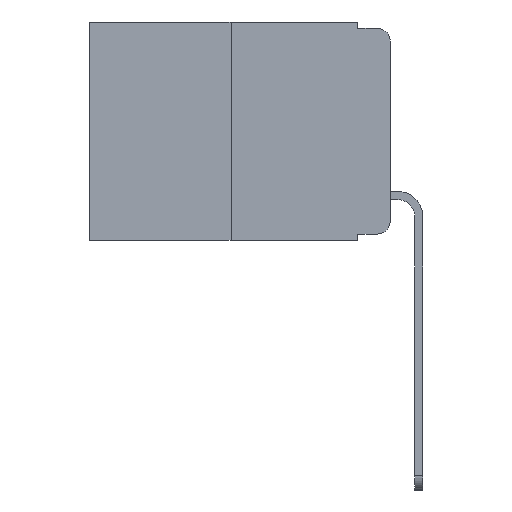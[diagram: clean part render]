
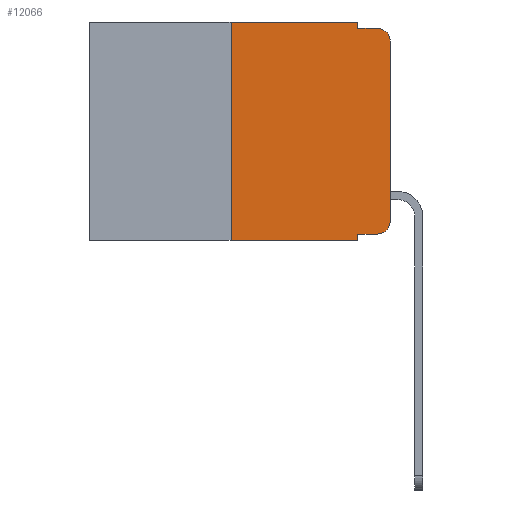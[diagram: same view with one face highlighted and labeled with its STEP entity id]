
A CAD part, left-side view. The second image highlights one B-rep face of the part: STEP entity #12066.
In plain terms, the highlighted planar face has unit normal (-1, 0, 0).
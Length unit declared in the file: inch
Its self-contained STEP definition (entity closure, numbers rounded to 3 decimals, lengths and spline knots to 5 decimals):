
#649 = VERTEX_POINT ( 'NONE', #21564 ) ;
#1145 = CARTESIAN_POINT ( 'NONE',  ( 0., 0.02, -0.03 ) ) ;
#1991 = DIRECTION ( 'NONE',  ( 0., -1., 0. ) ) ;
#2394 = EDGE_CURVE ( 'NONE', #15573, #7928, #8930, .T. ) ;
#2459 = ORIENTED_EDGE ( 'NONE', *, *, #2684, .T. ) ;
#2684 = EDGE_CURVE ( 'NONE', #18620, #20991, #10507, .T. ) ;
#2695 = ORIENTED_EDGE ( 'NONE', *, *, #24765, .T. ) ;
#3020 = CARTESIAN_POINT ( 'NONE',  ( 0., 0.02, -0.01 ) ) ;
#3289 = ORIENTED_EDGE ( 'NONE', *, *, #15235, .T. ) ;
#3310 = DIRECTION ( 'NONE',  ( 0., 0., -1. ) ) ;
#3337 = EDGE_CURVE ( 'NONE', #23345, #649, #3491, .T. ) ;
#3491 = LINE ( 'NONE', #7687, #9517 ) ;
#3604 = VERTEX_POINT ( 'NONE', #23397 ) ;
#3888 = DIRECTION ( 'NONE',  ( 0., 0., -1. ) ) ;
#4536 = LINE ( 'NONE', #23418, #25490 ) ;
#4589 = LINE ( 'NONE', #15803, #12536 ) ;
#7254 = EDGE_LOOP ( 'NONE', ( #25108, #21648, #25601, #14578, #23716, #25858, #3289, #10638, #2695, #2459 ) ) ;
#7653 = VERTEX_POINT ( 'NONE', #13378 ) ;
#7687 = CARTESIAN_POINT ( 'NONE',  ( 0., 0.473, 0. ) ) ;
#7928 = VERTEX_POINT ( 'NONE', #3020 ) ;
#8679 = CARTESIAN_POINT ( 'NONE',  ( 0., 0., -0.313 ) ) ;
#8694 = VECTOR ( 'NONE', #1991, 39.37008 ) ;
#8930 = CIRCLE ( 'NONE', #23483, 0.02 ) ;
#9517 = VECTOR ( 'NONE', #25947, 39.37008 ) ;
#10170 = LINE ( 'NONE', #23070, #24154 ) ;
#10470 = VECTOR ( 'NONE', #19628, 39.37008 ) ;
#10507 = CIRCLE ( 'NONE', #23189, 0.02 ) ;
#10638 = ORIENTED_EDGE ( 'NONE', *, *, #25176, .F. ) ;
#11068 = DIRECTION ( 'NONE',  ( 0., 0., -1. ) ) ;
#11239 = FACE_OUTER_BOUND ( 'NONE', #7254, .T. ) ;
#11242 = DIRECTION ( 'NONE',  ( 0., 0., -1. ) ) ;
#11667 = DIRECTION ( 'NONE',  ( 0., -1., 0. ) ) ;
#12066 = ADVANCED_FACE ( 'NONE', ( #11239 ), #17486, .F. ) ;
#12116 = CARTESIAN_POINT ( 'NONE',  ( 0., 0.02, -0.333 ) ) ;
#12536 = VECTOR ( 'NONE', #11667, 39.37008 ) ;
#12684 = LINE ( 'NONE', #15483, #10470 ) ;
#13378 = CARTESIAN_POINT ( 'NONE',  ( 0., 0.051, -0.01 ) ) ;
#14283 = AXIS2_PLACEMENT_3D ( 'NONE', #25680, #15438, #3310 ) ;
#14578 = ORIENTED_EDGE ( 'NONE', *, *, #15425, .F. ) ;
#15235 = EDGE_CURVE ( 'NONE', #3604, #19385, #10170, .T. ) ;
#15280 = EDGE_CURVE ( 'NONE', #3604, #23345, #17425, .T. ) ;
#15425 = EDGE_CURVE ( 'NONE', #649, #7653, #26030, .T. ) ;
#15438 = DIRECTION ( 'NONE',  ( 1., 0., 0. ) ) ;
#15470 = EDGE_CURVE ( 'NONE', #20991, #15573, #12684, .T. ) ;
#15483 = CARTESIAN_POINT ( 'NONE',  ( 0., 0., 0. ) ) ;
#15573 = VERTEX_POINT ( 'NONE', #18123 ) ;
#15803 = CARTESIAN_POINT ( 'NONE',  ( 0., 0.051, -0.01 ) ) ;
#15986 = DIRECTION ( 'NONE',  ( -1., 0., 0. ) ) ;
#17079 = CARTESIAN_POINT ( 'NONE',  ( 0., 0.25, 0. ) ) ;
#17425 = LINE ( 'NONE', #18848, #24123 ) ;
#17440 = DIRECTION ( 'NONE',  ( 0., 0., -1. ) ) ;
#17464 = CARTESIAN_POINT ( 'NONE',  ( 0., 0.051, -0.333 ) ) ;
#17486 = PLANE ( 'NONE',  #14283 ) ;
#17749 = VECTOR ( 'NONE', #17440, 39.37008 ) ;
#18123 = CARTESIAN_POINT ( 'NONE',  ( 0., 0., -0.03 ) ) ;
#18388 = EDGE_CURVE ( 'NONE', #7653, #7928, #4589, .T. ) ;
#18620 = VERTEX_POINT ( 'NONE', #12116 ) ;
#18848 = CARTESIAN_POINT ( 'NONE',  ( 0., 0.25, 0. ) ) ;
#19095 = DIRECTION ( 'NONE',  ( -1., 0., 0. ) ) ;
#19385 = VERTEX_POINT ( 'NONE', #20804 ) ;
#19628 = DIRECTION ( 'NONE',  ( 0., 0., 1. ) ) ;
#19967 = CARTESIAN_POINT ( 'NONE',  ( 0., 0.02, -0.313 ) ) ;
#20275 = CARTESIAN_POINT ( 'NONE',  ( 0., 0.051, -0.333 ) ) ;
#20804 = CARTESIAN_POINT ( 'NONE',  ( 0., 0.051, -0.343 ) ) ;
#20876 = DIRECTION ( 'NONE',  ( 0., 0., 1. ) ) ;
#20991 = VERTEX_POINT ( 'NONE', #8679 ) ;
#21564 = CARTESIAN_POINT ( 'NONE',  ( 0., 0.051, 0. ) ) ;
#21648 = ORIENTED_EDGE ( 'NONE', *, *, #2394, .T. ) ;
#23070 = CARTESIAN_POINT ( 'NONE',  ( 0., 0.473, -0.343 ) ) ;
#23189 = AXIS2_PLACEMENT_3D ( 'NONE', #19967, #15986, #3888 ) ;
#23345 = VERTEX_POINT ( 'NONE', #17079 ) ;
#23397 = CARTESIAN_POINT ( 'NONE',  ( 0., 0.25, -0.343 ) ) ;
#23418 = CARTESIAN_POINT ( 'NONE',  ( 0., 0.051, 0. ) ) ;
#23483 = AXIS2_PLACEMENT_3D ( 'NONE', #1145, #19095, #11068 ) ;
#23499 = CARTESIAN_POINT ( 'NONE',  ( 0., 0.051, 0. ) ) ;
#23716 = ORIENTED_EDGE ( 'NONE', *, *, #3337, .F. ) ;
#24123 = VECTOR ( 'NONE', #20876, 39.37008 ) ;
#24154 = VECTOR ( 'NONE', #24760, 39.37008 ) ;
#24760 = DIRECTION ( 'NONE',  ( 0., -1., 0. ) ) ;
#24765 = EDGE_CURVE ( 'NONE', #26189, #18620, #24886, .T. ) ;
#24886 = LINE ( 'NONE', #20275, #8694 ) ;
#25108 = ORIENTED_EDGE ( 'NONE', *, *, #15470, .T. ) ;
#25176 = EDGE_CURVE ( 'NONE', #26189, #19385, #4536, .T. ) ;
#25490 = VECTOR ( 'NONE', #11242, 39.37008 ) ;
#25601 = ORIENTED_EDGE ( 'NONE', *, *, #18388, .F. ) ;
#25680 = CARTESIAN_POINT ( 'NONE',  ( 0., 0.473, 0. ) ) ;
#25858 = ORIENTED_EDGE ( 'NONE', *, *, #15280, .F. ) ;
#25947 = DIRECTION ( 'NONE',  ( 0., -1., 0. ) ) ;
#26030 = LINE ( 'NONE', #23499, #17749 ) ;
#26189 = VERTEX_POINT ( 'NONE', #17464 ) ;
